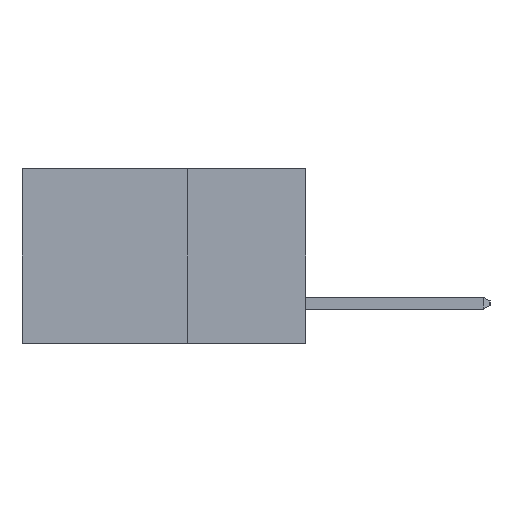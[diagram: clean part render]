
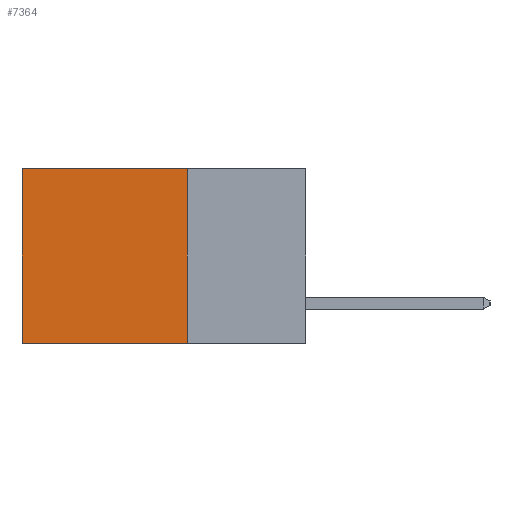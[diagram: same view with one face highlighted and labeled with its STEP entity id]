
A CAD part, left-side view. The second image highlights one B-rep face of the part: STEP entity #7364.
In plain terms, the highlighted planar face has unit normal (-1, 0, 0).
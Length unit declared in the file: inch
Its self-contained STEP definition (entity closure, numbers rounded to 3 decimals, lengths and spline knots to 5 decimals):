
#273 = LINE ( 'NONE', #10403, #7496 ) ;
#2146 = FACE_OUTER_BOUND ( 'NONE', #5927, .T. ) ;
#2612 = VECTOR ( 'NONE', #8767, 39.37008 ) ;
#2700 = DIRECTION ( 'NONE',  ( 0., 1., 0. ) ) ;
#2845 = VERTEX_POINT ( 'NONE', #7556 ) ;
#3070 = CARTESIAN_POINT ( 'NONE',  ( 0.298, 0.6, 0. ) ) ;
#3333 = VERTEX_POINT ( 'NONE', #10837 ) ;
#3690 = CARTESIAN_POINT ( 'NONE',  ( 0.298, 0.25, 0. ) ) ;
#3799 = LINE ( 'NONE', #3070, #5941 ) ;
#4164 = DIRECTION ( 'NONE',  ( 1., 0., 0. ) ) ;
#5475 = ORIENTED_EDGE ( 'NONE', *, *, #9723, .T. ) ;
#5874 = DIRECTION ( 'NONE',  ( 0., 0., -1. ) ) ;
#5927 = EDGE_LOOP ( 'NONE', ( #5475, #8590, #7275, #8088 ) ) ;
#5933 = CARTESIAN_POINT ( 'NONE',  ( 0.298, 0.25, 0. ) ) ;
#5941 = VECTOR ( 'NONE', #5874, 39.37008 ) ;
#6608 = VERTEX_POINT ( 'NONE', #6645 ) ;
#6645 = CARTESIAN_POINT ( 'NONE',  ( 0.298, 0.6, -0.37 ) ) ;
#7000 = VECTOR ( 'NONE', #2700, 39.37008 ) ;
#7275 = ORIENTED_EDGE ( 'NONE', *, *, #8571, .F. ) ;
#7364 = ADVANCED_FACE ( 'NONE', ( #2146 ), #9347, .F. ) ;
#7437 = CARTESIAN_POINT ( 'NONE',  ( 0.298, 0.6, 0. ) ) ;
#7496 = VECTOR ( 'NONE', #11229, 39.37008 ) ;
#7556 = CARTESIAN_POINT ( 'NONE',  ( 0.298, 0.25, -0.37 ) ) ;
#7981 = CARTESIAN_POINT ( 'NONE',  ( 0.298, 0.25, 0. ) ) ;
#8088 = ORIENTED_EDGE ( 'NONE', *, *, #11329, .T. ) ;
#8357 = AXIS2_PLACEMENT_3D ( 'NONE', #5933, #4164, #10176 ) ;
#8560 = EDGE_CURVE ( 'NONE', #2845, #6608, #273, .T. ) ;
#8571 = EDGE_CURVE ( 'NONE', #3333, #2845, #9682, .T. ) ;
#8590 = ORIENTED_EDGE ( 'NONE', *, *, #8560, .F. ) ;
#8767 = DIRECTION ( 'NONE',  ( 0., 0., -1. ) ) ;
#8842 = VERTEX_POINT ( 'NONE', #7437 ) ;
#9347 = PLANE ( 'NONE',  #8357 ) ;
#9682 = LINE ( 'NONE', #7981, #2612 ) ;
#9723 = EDGE_CURVE ( 'NONE', #8842, #6608, #3799, .T. ) ;
#10176 = DIRECTION ( 'NONE',  ( 0., 0., -1. ) ) ;
#10403 = CARTESIAN_POINT ( 'NONE',  ( 0.298, 0.25, -0.37 ) ) ;
#10837 = CARTESIAN_POINT ( 'NONE',  ( 0.298, 0.25, 0. ) ) ;
#11229 = DIRECTION ( 'NONE',  ( 0., 1., 0. ) ) ;
#11329 = EDGE_CURVE ( 'NONE', #3333, #8842, #11422, .T. ) ;
#11422 = LINE ( 'NONE', #3690, #7000 ) ;
